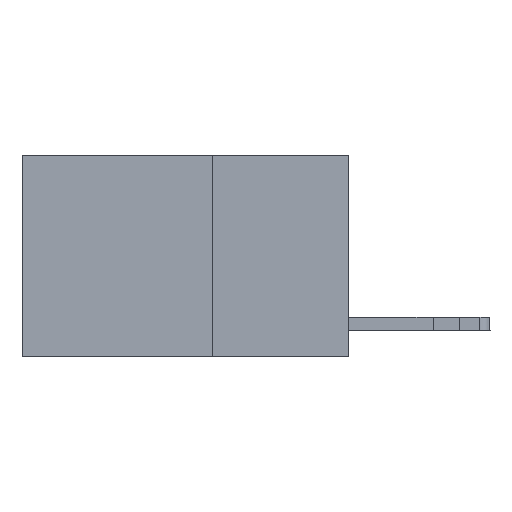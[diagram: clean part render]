
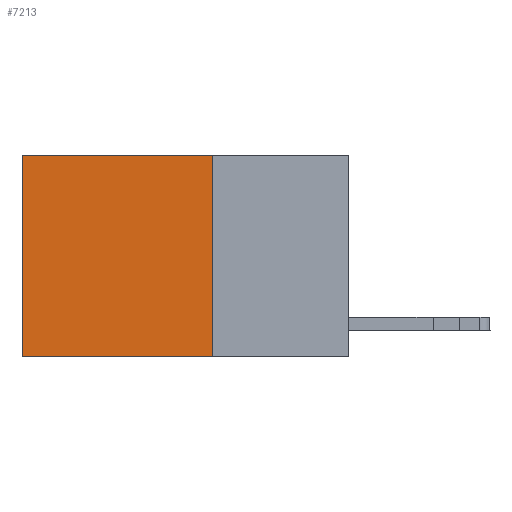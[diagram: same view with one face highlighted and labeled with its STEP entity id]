
A CAD part, left-side view. The second image highlights one B-rep face of the part: STEP entity #7213.
In plain terms, the highlighted planar face has unit normal (-1, 0, 0).
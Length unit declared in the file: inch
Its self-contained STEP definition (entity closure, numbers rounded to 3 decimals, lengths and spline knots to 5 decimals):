
#131 = DIRECTION ( 'NONE',  ( 0., 0., -1. ) ) ;
#242 = ORIENTED_EDGE ( 'NONE', *, *, #12208, .T. ) ;
#907 = VECTOR ( 'NONE', #14899, 39.37008 ) ;
#1251 = EDGE_CURVE ( 'NONE', #15776, #1956, #3658, .T. ) ;
#1425 = EDGE_CURVE ( 'NONE', #11558, #7984, #3900, .T. ) ;
#1956 = VERTEX_POINT ( 'NONE', #8131 ) ;
#2340 = PLANE ( 'NONE',  #9133 ) ;
#2414 = CARTESIAN_POINT ( 'NONE',  ( 0.2625, 0.25, 0. ) ) ;
#2420 = DIRECTION ( 'NONE',  ( 1., 0., 0. ) ) ;
#2460 = CARTESIAN_POINT ( 'NONE',  ( 0.2625, 0.6, -0.37 ) ) ;
#2727 = CARTESIAN_POINT ( 'NONE',  ( 0.2625, 0.6, 0. ) ) ;
#3658 = LINE ( 'NONE', #7430, #5268 ) ;
#3900 = LINE ( 'NONE', #8881, #12203 ) ;
#3931 = ORIENTED_EDGE ( 'NONE', *, *, #1251, .T. ) ;
#3947 = ORIENTED_EDGE ( 'NONE', *, *, #1425, .F. ) ;
#5268 = VECTOR ( 'NONE', #9814, 39.37008 ) ;
#7213 = ADVANCED_FACE ( 'NONE', ( #11195 ), #2340, .F. ) ;
#7430 = CARTESIAN_POINT ( 'NONE',  ( 0.2625, 0.25, 0. ) ) ;
#7593 = CARTESIAN_POINT ( 'NONE',  ( 0.2625, 0.25, 0. ) ) ;
#7984 = VERTEX_POINT ( 'NONE', #2460 ) ;
#8131 = CARTESIAN_POINT ( 'NONE',  ( 0.2625, 0.6, 0. ) ) ;
#8395 = CARTESIAN_POINT ( 'NONE',  ( 0.2625, 0.25, -0.37 ) ) ;
#8881 = CARTESIAN_POINT ( 'NONE',  ( 0.2625, 0.25, -0.37 ) ) ;
#9133 = AXIS2_PLACEMENT_3D ( 'NONE', #7593, #2420, #131 ) ;
#9803 = CARTESIAN_POINT ( 'NONE',  ( 0.2625, 0.25, 0. ) ) ;
#9814 = DIRECTION ( 'NONE',  ( 0., 1., 0. ) ) ;
#9883 = LINE ( 'NONE', #9803, #907 ) ;
#10334 = DIRECTION ( 'NONE',  ( 0., 0., -1. ) ) ;
#11195 = FACE_OUTER_BOUND ( 'NONE', #13083, .T. ) ;
#11242 = LINE ( 'NONE', #2727, #14772 ) ;
#11558 = VERTEX_POINT ( 'NONE', #8395 ) ;
#12203 = VECTOR ( 'NONE', #13917, 39.37008 ) ;
#12208 = EDGE_CURVE ( 'NONE', #1956, #7984, #11242, .T. ) ;
#13083 = EDGE_LOOP ( 'NONE', ( #242, #3947, #14643, #3931 ) ) ;
#13917 = DIRECTION ( 'NONE',  ( 0., 1., 0. ) ) ;
#14643 = ORIENTED_EDGE ( 'NONE', *, *, #14651, .F. ) ;
#14651 = EDGE_CURVE ( 'NONE', #15776, #11558, #9883, .T. ) ;
#14772 = VECTOR ( 'NONE', #10334, 39.37008 ) ;
#14899 = DIRECTION ( 'NONE',  ( 0., 0., -1. ) ) ;
#15776 = VERTEX_POINT ( 'NONE', #2414 ) ;
